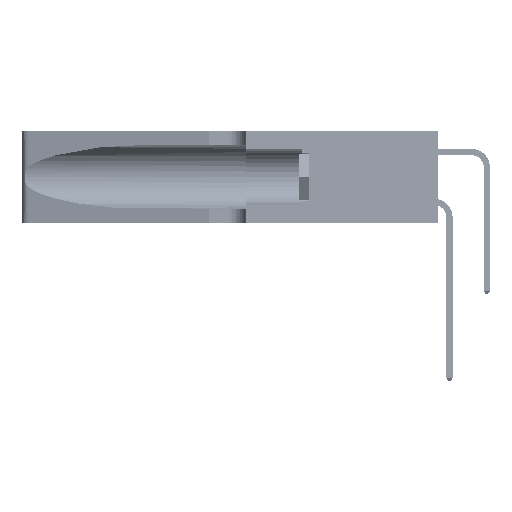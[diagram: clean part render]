
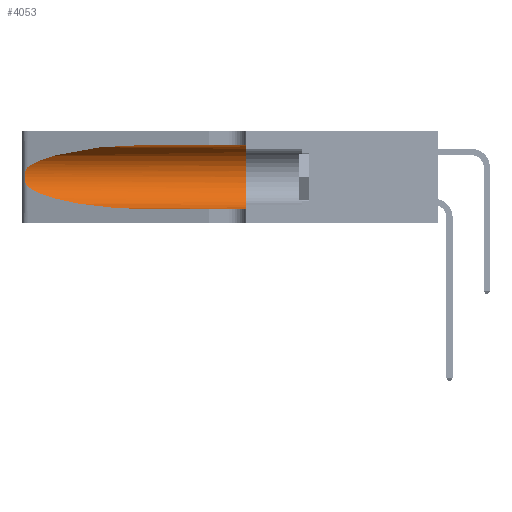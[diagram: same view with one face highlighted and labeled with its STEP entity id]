
A CAD part, left-side view. The second image highlights one B-rep face of the part: STEP entity #4053.
In plain terms, the highlighted cylindrical face has radius 3.308 mm (diameter 6.617 mm), a partial arc.
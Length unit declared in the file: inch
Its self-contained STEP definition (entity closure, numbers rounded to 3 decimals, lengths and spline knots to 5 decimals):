
#200 = CARTESIAN_POINT ( 'NONE',  ( 0.1305, 0.35, 0.05475 ) ) ;
#868 = ORIENTED_EDGE ( 'NONE', *, *, #37757, .F. ) ;
#963 = CARTESIAN_POINT ( 'NONE',  ( 0.25854, 1.2359, 0.20912 ) ) ;
#1667 = B_SPLINE_CURVE_WITH_KNOTS ( 'NONE', 3,
 ( #47188, #4683, #39521, #24225, #963, #28099, #4841, #31973, #8759, #35852, #12723, #39688, #16598, #43543 ),
 .UNSPECIFIED., .F., .F.,
 ( 4, 2, 2, 2, 2, 2, 4 ),
 ( 0., 0.00027, 0.00053, 0.00107, 0.0016, 0.00187, 0.00214 ),
 .UNSPECIFIED. ) ;
#2609 = CARTESIAN_POINT ( 'NONE',  ( 0.1305, 1.61858, 0.05475 ) ) ;
#2668 = ORIENTED_EDGE ( 'NONE', *, *, #47918, .T. ) ;
#4053 = ADVANCED_FACE ( 'NONE', ( #15264 ), #44777, .F. ) ;
#4683 = CARTESIAN_POINT ( 'NONE',  ( 0.25555, 1.22994, 0.2215 ) ) ;
#4841 = CARTESIAN_POINT ( 'NONE',  ( 0.26075, 1.23896, 0.19203 ) ) ;
#5179 = DIRECTION ( 'NONE',  ( 0., -1., 0. ) ) ;
#6305 = EDGE_CURVE ( 'NONE', #15043, #15035, #9942, .T. ) ;
#6914 =( BOUNDED_CURVE ( )  B_SPLINE_CURVE ( 3, ( #24006, #27878, #8543, #35629 ),
 .UNSPECIFIED., .F., .F. ) 
 B_SPLINE_CURVE_WITH_KNOTS ( ( 4, 4 ),
 ( 1.5708, 2.84003 ),
 .UNSPECIFIED. ) 
 CURVE ( )  GEOMETRIC_REPRESENTATION_ITEM ( )  RATIONAL_B_SPLINE_CURVE ( ( 1., 0.87, 0.87, 1. ) ) 
 REPRESENTATION_ITEM ( '' )  );
#7842 = LINE ( 'NONE', #2609, #38694 ) ;
#8543 = CARTESIAN_POINT ( 'NONE',  ( 0.2373, 1.15595, 0.28018 ) ) ;
#8759 = CARTESIAN_POINT ( 'NONE',  ( 0.26017, 1.23833, 0.17102 ) ) ;
#9109 = CARTESIAN_POINT ( 'NONE',  ( 0.1305, 1.61858, 0.185 ) ) ;
#9942 = LINE ( 'NONE', #42785, #11169 ) ;
#10542 = CARTESIAN_POINT ( 'NONE',  ( 0.1305, 0.72297, 0.05475 ) ) ;
#11169 = VECTOR ( 'NONE', #19757, 39.37008 ) ;
#12582 = VERTEX_POINT ( 'NONE', #200 ) ;
#12723 = CARTESIAN_POINT ( 'NONE',  ( 0.25789, 1.23486, 0.15765 ) ) ;
#14008 = EDGE_CURVE ( 'NONE', #36562, #22329, #1667, .T. ) ;
#14149 = VERTEX_POINT ( 'NONE', #36856 ) ;
#15035 = VERTEX_POINT ( 'NONE', #19488 ) ;
#15043 = VERTEX_POINT ( 'NONE', #42501 ) ;
#15264 = FACE_OUTER_BOUND ( 'NONE', #49026, .T. ) ;
#16598 = CARTESIAN_POINT ( 'NONE',  ( 0.25555, 1.22993, 0.14849 ) ) ;
#17950 = DIRECTION ( 'NONE',  ( 0., 1., 0. ) ) ;
#19488 = CARTESIAN_POINT ( 'NONE',  ( 0.1305, 0.35, 0.31525 ) ) ;
#19757 = DIRECTION ( 'NONE',  ( 0., -1., 0. ) ) ;
#20313 = AXIS2_PLACEMENT_3D ( 'NONE', #9109, #5179, #32290 ) ;
#21313 = ORIENTED_EDGE ( 'NONE', *, *, #6305, .F. ) ;
#22100 = CIRCLE ( 'NONE', #36927, 0.13025 ) ;
#22106 = CARTESIAN_POINT ( 'NONE',  ( 0.2373, 1.15595, 0.08982 ) ) ;
#22329 = VERTEX_POINT ( 'NONE', #26655 ) ;
#23417 = EDGE_CURVE ( 'NONE', #14149, #12582, #7842, .T. ) ;
#24006 = CARTESIAN_POINT ( 'NONE',  ( 0.1305, 0.72297, 0.31525 ) ) ;
#24225 = CARTESIAN_POINT ( 'NONE',  ( 0.25787, 1.23484, 0.2124 ) ) ;
#26655 = CARTESIAN_POINT ( 'NONE',  ( 0.25487, 1.22718, 0.14631 ) ) ;
#27878 = CARTESIAN_POINT ( 'NONE',  ( 0.18966, 0.96281, 0.31525 ) ) ;
#28099 = CARTESIAN_POINT ( 'NONE',  ( 0.26018, 1.23835, 0.19895 ) ) ;
#28312 = ORIENTED_EDGE ( 'NONE', *, *, #36100, .T. ) ;
#29732 = DIRECTION ( 'NONE',  ( 0., -1., 0. ) ) ;
#31973 = CARTESIAN_POINT ( 'NONE',  ( 0.26075, 1.23896, 0.178 ) ) ;
#32290 = DIRECTION ( 'NONE',  ( 0., 0., -1. ) ) ;
#33717 = CARTESIAN_POINT ( 'NONE',  ( 0.18966, 0.96281, 0.05475 ) ) ;
#35629 = CARTESIAN_POINT ( 'NONE',  ( 0.25487, 1.22718, 0.22369 ) ) ;
#35852 = CARTESIAN_POINT ( 'NONE',  ( 0.25856, 1.23593, 0.16098 ) ) ;
#36100 = EDGE_CURVE ( 'NONE', #15043, #36562, #6914, .T. ) ;
#36562 = VERTEX_POINT ( 'NONE', #45933 ) ;
#36856 = CARTESIAN_POINT ( 'NONE',  ( 0.1305, 0.72297, 0.05475 ) ) ;
#36927 = AXIS2_PLACEMENT_3D ( 'NONE', #41021, #17950, #44852 ) ;
#37757 = EDGE_CURVE ( 'NONE', #15035, #12582, #22100, .T. ) ;
#38694 = VECTOR ( 'NONE', #29732, 39.37008 ) ;
#39521 = CARTESIAN_POINT ( 'NONE',  ( 0.25639, 1.23184, 0.21858 ) ) ;
#39688 = CARTESIAN_POINT ( 'NONE',  ( 0.25639, 1.23186, 0.15144 ) ) ;
#41021 = CARTESIAN_POINT ( 'NONE',  ( 0.1305, 0.35, 0.185 ) ) ;
#42501 = CARTESIAN_POINT ( 'NONE',  ( 0.1305, 0.72297, 0.31525 ) ) ;
#42785 = CARTESIAN_POINT ( 'NONE',  ( 0.1305, 1.61858, 0.31525 ) ) ;
#43543 = CARTESIAN_POINT ( 'NONE',  ( 0.25487, 1.22718, 0.14631 ) ) ;
#44393 =( BOUNDED_CURVE ( )  B_SPLINE_CURVE ( 3, ( #48893, #22106, #33717, #10542 ),
 .UNSPECIFIED., .F., .F. ) 
 B_SPLINE_CURVE_WITH_KNOTS ( ( 4, 4 ),
 ( 3.44316, 4.71239 ),
 .UNSPECIFIED. ) 
 CURVE ( )  GEOMETRIC_REPRESENTATION_ITEM ( )  RATIONAL_B_SPLINE_CURVE ( ( 1., 0.87, 0.87, 1. ) ) 
 REPRESENTATION_ITEM ( '' )  );
#44777 = CYLINDRICAL_SURFACE ( 'NONE', #20313, 0.13025 ) ;
#44852 = DIRECTION ( 'NONE',  ( 0., 0., 1. ) ) ;
#45537 = ORIENTED_EDGE ( 'NONE', *, *, #14008, .T. ) ;
#45933 = CARTESIAN_POINT ( 'NONE',  ( 0.25487, 1.22718, 0.22369 ) ) ;
#47188 = CARTESIAN_POINT ( 'NONE',  ( 0.25487, 1.22718, 0.22369 ) ) ;
#47918 = EDGE_CURVE ( 'NONE', #22329, #14149, #44393, .T. ) ;
#48539 = ORIENTED_EDGE ( 'NONE', *, *, #23417, .T. ) ;
#48893 = CARTESIAN_POINT ( 'NONE',  ( 0.25487, 1.22718, 0.14631 ) ) ;
#49026 = EDGE_LOOP ( 'NONE', ( #28312, #45537, #2668, #48539, #868, #21313 ) ) ;
